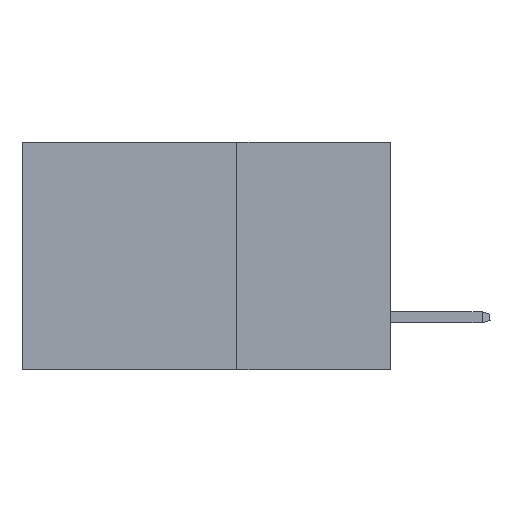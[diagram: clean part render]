
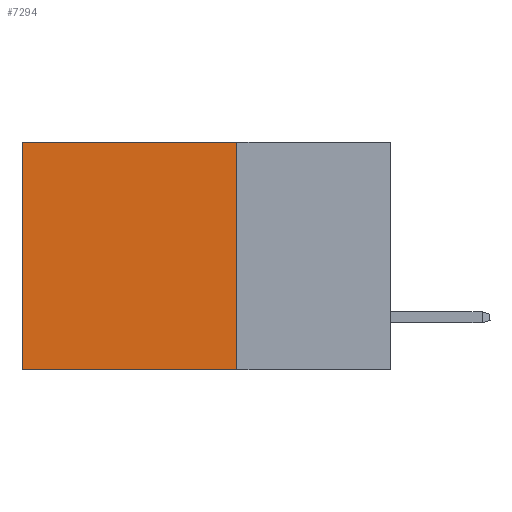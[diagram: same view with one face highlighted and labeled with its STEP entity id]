
A CAD part, left-side view. The second image highlights one B-rep face of the part: STEP entity #7294.
In plain terms, the highlighted planar face has unit normal (-1, 0, 0).
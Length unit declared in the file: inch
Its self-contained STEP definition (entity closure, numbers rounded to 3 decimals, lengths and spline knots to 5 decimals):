
#334 = DIRECTION ( 'NONE',  ( 0., 0., -1. ) ) ;
#354 = VERTEX_POINT ( 'NONE', #11056 ) ;
#1726 = VECTOR ( 'NONE', #12607, 39.37008 ) ;
#3590 = ORIENTED_EDGE ( 'NONE', *, *, #10053, .F. ) ;
#3766 = CARTESIAN_POINT ( 'NONE',  ( 0.2875, 0.25, 0. ) ) ;
#3828 = VECTOR ( 'NONE', #5862, 39.37008 ) ;
#4079 = VERTEX_POINT ( 'NONE', #4285 ) ;
#4285 = CARTESIAN_POINT ( 'NONE',  ( 0.2875, 0.6, 0. ) ) ;
#4437 = FACE_OUTER_BOUND ( 'NONE', #6836, .T. ) ;
#4813 = DIRECTION ( 'NONE',  ( 1., 0., 0. ) ) ;
#4821 = CARTESIAN_POINT ( 'NONE',  ( 0.2875, 0.25, -0.37 ) ) ;
#5336 = CARTESIAN_POINT ( 'NONE',  ( 0.2875, 0.25, -0.37 ) ) ;
#5478 = ORIENTED_EDGE ( 'NONE', *, *, #5860, .F. ) ;
#5676 = VERTEX_POINT ( 'NONE', #8681 ) ;
#5860 = EDGE_CURVE ( 'NONE', #8207, #354, #9377, .T. ) ;
#5862 = DIRECTION ( 'NONE',  ( 0., 1., 0. ) ) ;
#6645 = EDGE_CURVE ( 'NONE', #5676, #4079, #6747, .T. ) ;
#6747 = LINE ( 'NONE', #13259, #9185 ) ;
#6836 = EDGE_LOOP ( 'NONE', ( #11842, #5478, #3590, #12863 ) ) ;
#7263 = AXIS2_PLACEMENT_3D ( 'NONE', #3766, #4813, #12067 ) ;
#7294 = ADVANCED_FACE ( 'NONE', ( #4437 ), #9990, .F. ) ;
#8080 = DIRECTION ( 'NONE',  ( 0., 1., 0. ) ) ;
#8207 = VERTEX_POINT ( 'NONE', #5336 ) ;
#8681 = CARTESIAN_POINT ( 'NONE',  ( 0.2875, 0.25, 0. ) ) ;
#9185 = VECTOR ( 'NONE', #8080, 39.37008 ) ;
#9377 = LINE ( 'NONE', #4821, #3828 ) ;
#9990 = PLANE ( 'NONE',  #7263 ) ;
#10019 = LINE ( 'NONE', #11560, #1726 ) ;
#10053 = EDGE_CURVE ( 'NONE', #5676, #8207, #10019, .T. ) ;
#11056 = CARTESIAN_POINT ( 'NONE',  ( 0.2875, 0.6, -0.37 ) ) ;
#11560 = CARTESIAN_POINT ( 'NONE',  ( 0.2875, 0.25, 0. ) ) ;
#11842 = ORIENTED_EDGE ( 'NONE', *, *, #12124, .T. ) ;
#12067 = DIRECTION ( 'NONE',  ( 0., 0., -1. ) ) ;
#12124 = EDGE_CURVE ( 'NONE', #4079, #354, #12557, .T. ) ;
#12227 = VECTOR ( 'NONE', #334, 39.37008 ) ;
#12557 = LINE ( 'NONE', #12788, #12227 ) ;
#12607 = DIRECTION ( 'NONE',  ( 0., 0., -1. ) ) ;
#12788 = CARTESIAN_POINT ( 'NONE',  ( 0.2875, 0.6, 0. ) ) ;
#12863 = ORIENTED_EDGE ( 'NONE', *, *, #6645, .T. ) ;
#13259 = CARTESIAN_POINT ( 'NONE',  ( 0.2875, 0.25, 0. ) ) ;
